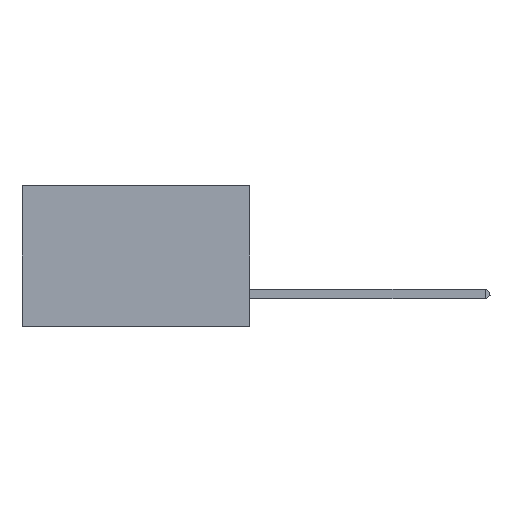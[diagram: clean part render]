
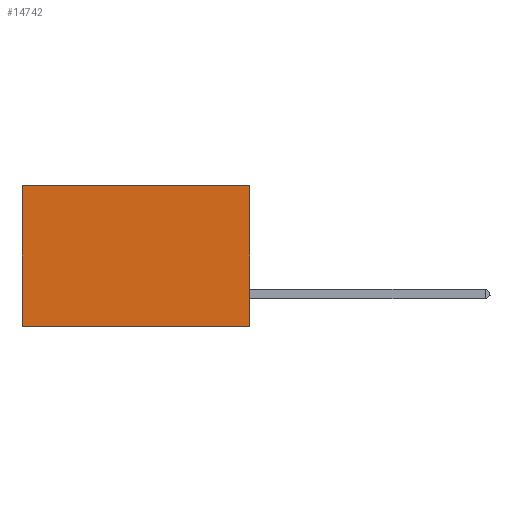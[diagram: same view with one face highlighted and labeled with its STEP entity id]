
A CAD part, left-side view. The second image highlights one B-rep face of the part: STEP entity #14742.
In plain terms, the highlighted planar face has unit normal (-1, 0, 0).
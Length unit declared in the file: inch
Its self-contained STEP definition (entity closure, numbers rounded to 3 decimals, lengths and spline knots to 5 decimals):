
#1992 = VECTOR ( 'NONE', #12753, 39.37008 ) ;
#2747 = VERTEX_POINT ( 'NONE', #7773 ) ;
#3416 = VECTOR ( 'NONE', #6342, 39.37008 ) ;
#3821 = ORIENTED_EDGE ( 'NONE', *, *, #5468, .F. ) ;
#4997 = ORIENTED_EDGE ( 'NONE', *, *, #23070, .F. ) ;
#5031 = CARTESIAN_POINT ( 'NONE',  ( 0.2875, 0., 0. ) ) ;
#5468 = EDGE_CURVE ( 'NONE', #9113, #16302, #14091, .T. ) ;
#5748 = VECTOR ( 'NONE', #17186, 39.37008 ) ;
#5827 = CARTESIAN_POINT ( 'NONE',  ( 0.2875, 0., 0. ) ) ;
#5996 = EDGE_CURVE ( 'NONE', #2747, #16302, #20884, .T. ) ;
#6342 = DIRECTION ( 'NONE',  ( 0., 1., 0. ) ) ;
#7668 = ORIENTED_EDGE ( 'NONE', *, *, #5996, .T. ) ;
#7773 = CARTESIAN_POINT ( 'NONE',  ( 0.2875, 0.6, 0. ) ) ;
#7800 = AXIS2_PLACEMENT_3D ( 'NONE', #11882, #7909, #23267 ) ;
#7909 = DIRECTION ( 'NONE',  ( 1., 0., 0. ) ) ;
#7922 = LINE ( 'NONE', #5031, #1992 ) ;
#9113 = VERTEX_POINT ( 'NONE', #17149 ) ;
#9443 = VECTOR ( 'NONE', #13449, 39.37008 ) ;
#9859 = CARTESIAN_POINT ( 'NONE',  ( 0.2875, 0.6, 0. ) ) ;
#10038 = LINE ( 'NONE', #5827, #9443 ) ;
#11339 = EDGE_CURVE ( 'NONE', #15608, #2747, #10038, .T. ) ;
#11850 = CARTESIAN_POINT ( 'NONE',  ( 0.2875, 0., 0. ) ) ;
#11882 = CARTESIAN_POINT ( 'NONE',  ( 0.2875, 0., 0. ) ) ;
#12753 = DIRECTION ( 'NONE',  ( 0., 0., -1. ) ) ;
#13360 = EDGE_LOOP ( 'NONE', ( #7668, #3821, #4997, #16441 ) ) ;
#13449 = DIRECTION ( 'NONE',  ( 0., 1., 0. ) ) ;
#14091 = LINE ( 'NONE', #16000, #3416 ) ;
#14742 = ADVANCED_FACE ( 'NONE', ( #17827 ), #15641, .F. ) ;
#15608 = VERTEX_POINT ( 'NONE', #11850 ) ;
#15641 = PLANE ( 'NONE',  #7800 ) ;
#16000 = CARTESIAN_POINT ( 'NONE',  ( 0.2875, 0., -0.37 ) ) ;
#16100 = CARTESIAN_POINT ( 'NONE',  ( 0.2875, 0.6, -0.37 ) ) ;
#16302 = VERTEX_POINT ( 'NONE', #16100 ) ;
#16441 = ORIENTED_EDGE ( 'NONE', *, *, #11339, .T. ) ;
#17149 = CARTESIAN_POINT ( 'NONE',  ( 0.2875, 0., -0.37 ) ) ;
#17186 = DIRECTION ( 'NONE',  ( 0., 0., -1. ) ) ;
#17827 = FACE_OUTER_BOUND ( 'NONE', #13360, .T. ) ;
#20884 = LINE ( 'NONE', #9859, #5748 ) ;
#23070 = EDGE_CURVE ( 'NONE', #15608, #9113, #7922, .T. ) ;
#23267 = DIRECTION ( 'NONE',  ( 0., 0., -1. ) ) ;
